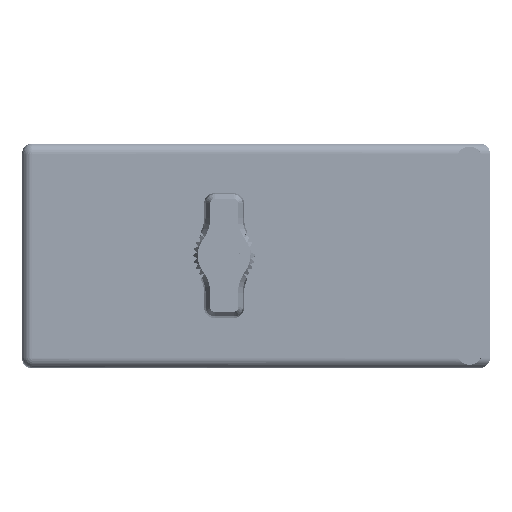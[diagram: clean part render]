
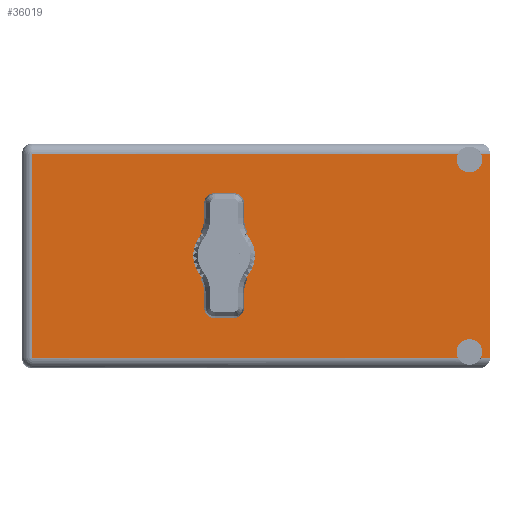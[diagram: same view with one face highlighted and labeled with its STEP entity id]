
A CAD part, top view. The second image highlights one B-rep face of the part: STEP entity #36019.
In plain terms, the highlighted face is planar.
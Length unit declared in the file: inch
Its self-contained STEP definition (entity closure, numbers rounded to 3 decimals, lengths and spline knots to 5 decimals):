
#2694 = AXIS2_PLACEMENT_3D ( 'NONE', #80097, #72002, #80494 ) ;
#6304 = CARTESIAN_POINT ( 'NONE',  ( 3.05, 2.03, -1.421 ) ) ;
#8431 = DIRECTION ( 'NONE',  ( 1., 0., 0. ) ) ;
#9625 = CARTESIAN_POINT ( 'NONE',  ( 3.19, 2.03, -0.07 ) ) ;
#10237 = VECTOR ( 'NONE', #64634, 39.37008 ) ;
#12753 = ORIENTED_EDGE ( 'NONE', *, *, #66222, .T. ) ;
#13736 = DIRECTION ( 'NONE',  ( 0., 0., 1. ) ) ;
#13952 = CARTESIAN_POINT ( 'NONE',  ( 3.19, 2.03, -0.07 ) ) ;
#14563 = DIRECTION ( 'NONE',  ( 0., 0., 1. ) ) ;
#14750 = EDGE_CURVE ( 'NONE', #107807, #82213, #61761, .T. ) ;
#14851 = VERTEX_POINT ( 'NONE', #44700 ) ;
#15225 = DIRECTION ( 'NONE',  ( 0., 0., 1. ) ) ;
#16040 = DIRECTION ( 'NONE',  ( 0., 1., 0. ) ) ;
#16216 = LINE ( 'NONE', #59839, #110960 ) ;
#20291 = VERTEX_POINT ( 'NONE', #67401 ) ;
#23142 = VERTEX_POINT ( 'NONE', #94304 ) ;
#23155 = ORIENTED_EDGE ( 'NONE', *, *, #91609, .T. ) ;
#23713 = FACE_BOUND ( 'NONE', #48212, .T. ) ;
#24459 = DIRECTION ( 'NONE',  ( 0., 1., 0. ) ) ;
#25725 = AXIS2_PLACEMENT_3D ( 'NONE', #6304, #89287, #108943 ) ;
#26713 = CARTESIAN_POINT ( 'NONE',  ( 0.07, 2.03, -0.07 ) ) ;
#29336 = CARTESIAN_POINT ( 'NONE',  ( 0., 2.03, -1.46 ) ) ;
#30397 = CARTESIAN_POINT ( 'NONE',  ( 0., 2.03, -1.53 ) ) ;
#31169 = CARTESIAN_POINT ( 'NONE',  ( 3.05, 2.03, -0.1965 ) ) ;
#32462 = CARTESIAN_POINT ( 'NONE',  ( 3.05, 2.03, -0.109 ) ) ;
#33725 = CIRCLE ( 'NONE', #38558, 0.17 ) ;
#35412 = CIRCLE ( 'NONE', #51645, 0.17 ) ;
#35854 = CARTESIAN_POINT ( 'NONE',  ( 2.97167, 2.03, -1.46 ) ) ;
#36019 = ADVANCED_FACE ( 'NONE', ( #23713, #102748 ), #113869, .T. ) ;
#38558 = AXIS2_PLACEMENT_3D ( 'NONE', #86766, #113261, #13736 ) ;
#39460 = ORIENTED_EDGE ( 'NONE', *, *, #50762, .T. ) ;
#40239 = DIRECTION ( 'NONE',  ( 0., 0., 1. ) ) ;
#41580 = DIRECTION ( 'NONE',  ( 1., 0., 0. ) ) ;
#42307 = VECTOR ( 'NONE', #58188, 39.37008 ) ;
#42447 = EDGE_CURVE ( 'NONE', #109914, #20291, #35412, .T. ) ;
#44700 = CARTESIAN_POINT ( 'NONE',  ( 0.07, 2.03, -1.46 ) ) ;
#48212 = EDGE_LOOP ( 'NONE', ( #107281, #87278 ) ) ;
#49567 = VECTOR ( 'NONE', #100696, 39.37008 ) ;
#50255 = EDGE_CURVE ( 'NONE', #53464, #97891, #53158, .T. ) ;
#50762 = EDGE_CURVE ( 'NONE', #107807, #117527, #67350, .T. ) ;
#50931 = VERTEX_POINT ( 'NONE', #35854 ) ;
#51139 = CARTESIAN_POINT ( 'NONE',  ( 3.19, 2.03, -0.07 ) ) ;
#51547 = VECTOR ( 'NONE', #8431, 39.37008 ) ;
#51645 = AXIS2_PLACEMENT_3D ( 'NONE', #75249, #68331, #40239 ) ;
#52120 = CIRCLE ( 'NONE', #99659, 0.0875 ) ;
#53158 = LINE ( 'NONE', #111229, #10237 ) ;
#53464 = VERTEX_POINT ( 'NONE', #115985 ) ;
#54096 = CARTESIAN_POINT ( 'NONE',  ( 3.12833, 2.03, -0.07 ) ) ;
#56515 = CARTESIAN_POINT ( 'NONE',  ( 1.3775, 2.03, -0.935 ) ) ;
#58188 = DIRECTION ( 'NONE',  ( -1., 0., 0. ) ) ;
#59217 = EDGE_CURVE ( 'NONE', #50931, #14851, #66694, .T. ) ;
#59839 = CARTESIAN_POINT ( 'NONE',  ( 3.19, 2.03, 0. ) ) ;
#61761 = CIRCLE ( 'NONE', #2694, 0.0875 ) ;
#63131 = ORIENTED_EDGE ( 'NONE', *, *, #59217, .T. ) ;
#64634 = DIRECTION ( 'NONE',  ( -1., 0., 0. ) ) ;
#66222 = EDGE_CURVE ( 'NONE', #96302, #75654, #105670, .T. ) ;
#66694 = LINE ( 'NONE', #29336, #42307 ) ;
#67350 = LINE ( 'NONE', #9625, #51547 ) ;
#67401 = CARTESIAN_POINT ( 'NONE',  ( 1.3775, 2.03, -0.595 ) ) ;
#68178 = EDGE_CURVE ( 'NONE', #53464, #117527, #16216, .T. ) ;
#68331 = DIRECTION ( 'NONE',  ( 0., 1., 0. ) ) ;
#69692 = ORIENTED_EDGE ( 'NONE', *, *, #50255, .T. ) ;
#69700 = VECTOR ( 'NONE', #41580, 39.37008 ) ;
#72002 = DIRECTION ( 'NONE',  ( 0., 1., 0. ) ) ;
#75249 = CARTESIAN_POINT ( 'NONE',  ( 1.3775, 2.03, -0.765 ) ) ;
#75654 = VERTEX_POINT ( 'NONE', #115627 ) ;
#80097 = CARTESIAN_POINT ( 'NONE',  ( 3.05, 2.03, -0.109 ) ) ;
#80494 = DIRECTION ( 'NONE',  ( 0., 0., 1. ) ) ;
#82213 = VERTEX_POINT ( 'NONE', #31169 ) ;
#82276 = CIRCLE ( 'NONE', #86440, 0.0875 ) ;
#82586 = CARTESIAN_POINT ( 'NONE',  ( 0.07, 2.03, -1.53 ) ) ;
#83237 = ORIENTED_EDGE ( 'NONE', *, *, #68178, .F. ) ;
#84997 = DIRECTION ( 'NONE',  ( 0., 0., 1. ) ) ;
#86440 = AXIS2_PLACEMENT_3D ( 'NONE', #89843, #16040, #15225 ) ;
#86632 = CARTESIAN_POINT ( 'NONE',  ( 3.12833, 2.03, -1.46 ) ) ;
#86766 = CARTESIAN_POINT ( 'NONE',  ( 1.3775, 2.03, -0.765 ) ) ;
#87278 = ORIENTED_EDGE ( 'NONE', *, *, #42447, .F. ) ;
#88040 = EDGE_CURVE ( 'NONE', #50931, #23142, #117641, .T. ) ;
#88293 = DIRECTION ( 'NONE',  ( 0., 0., 1. ) ) ;
#89287 = DIRECTION ( 'NONE',  ( 0., 1., 0. ) ) ;
#89843 = CARTESIAN_POINT ( 'NONE',  ( 3.05, 2.03, -1.421 ) ) ;
#91609 = EDGE_CURVE ( 'NONE', #14851, #96302, #105622, .T. ) ;
#92912 = ORIENTED_EDGE ( 'NONE', *, *, #88040, .F. ) ;
#94304 = CARTESIAN_POINT ( 'NONE',  ( 3.05, 2.03, -1.3335 ) ) ;
#94651 = DIRECTION ( 'NONE',  ( 0., 1., 0. ) ) ;
#95242 = ORIENTED_EDGE ( 'NONE', *, *, #104289, .F. ) ;
#96302 = VERTEX_POINT ( 'NONE', #26713 ) ;
#97891 = VERTEX_POINT ( 'NONE', #86632 ) ;
#99659 = AXIS2_PLACEMENT_3D ( 'NONE', #32462, #24459, #88293 ) ;
#100696 = DIRECTION ( 'NONE',  ( 0., 0., 1. ) ) ;
#102318 = EDGE_LOOP ( 'NONE', ( #12753, #114004, #112702, #39460, #83237, #69692, #95242, #92912, #63131, #23155 ) ) ;
#102748 = FACE_OUTER_BOUND ( 'NONE', #102318, .T. ) ;
#104289 = EDGE_CURVE ( 'NONE', #23142, #97891, #82276, .T. ) ;
#105622 = LINE ( 'NONE', #82586, #49567 ) ;
#105670 = LINE ( 'NONE', #13952, #69700 ) ;
#107281 = ORIENTED_EDGE ( 'NONE', *, *, #111958, .F. ) ;
#107807 = VERTEX_POINT ( 'NONE', #54096 ) ;
#108943 = DIRECTION ( 'NONE',  ( 0., 0., 1. ) ) ;
#109914 = VERTEX_POINT ( 'NONE', #56515 ) ;
#110448 = AXIS2_PLACEMENT_3D ( 'NONE', #30397, #94651, #84997 ) ;
#110960 = VECTOR ( 'NONE', #14563, 39.37008 ) ;
#111229 = CARTESIAN_POINT ( 'NONE',  ( 0., 2.03, -1.46 ) ) ;
#111958 = EDGE_CURVE ( 'NONE', #20291, #109914, #33725, .T. ) ;
#112702 = ORIENTED_EDGE ( 'NONE', *, *, #14750, .F. ) ;
#113261 = DIRECTION ( 'NONE',  ( 0., 1., 0. ) ) ;
#113869 = PLANE ( 'NONE',  #110448 ) ;
#114004 = ORIENTED_EDGE ( 'NONE', *, *, #116699, .F. ) ;
#115627 = CARTESIAN_POINT ( 'NONE',  ( 2.97167, 2.03, -0.07 ) ) ;
#115985 = CARTESIAN_POINT ( 'NONE',  ( 3.19, 2.03, -1.46 ) ) ;
#116699 = EDGE_CURVE ( 'NONE', #82213, #75654, #52120, .T. ) ;
#117527 = VERTEX_POINT ( 'NONE', #51139 ) ;
#117641 = CIRCLE ( 'NONE', #25725, 0.0875 ) ;
